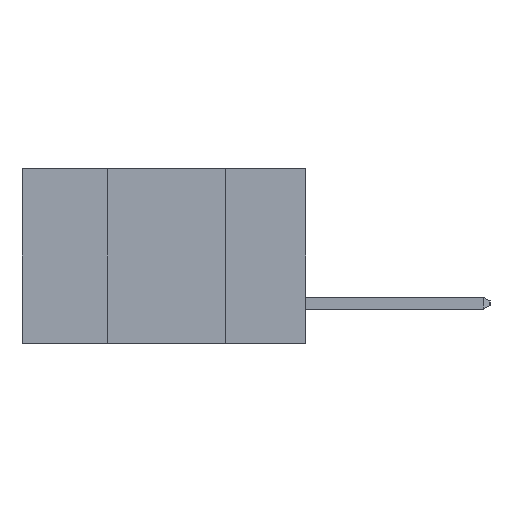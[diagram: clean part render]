
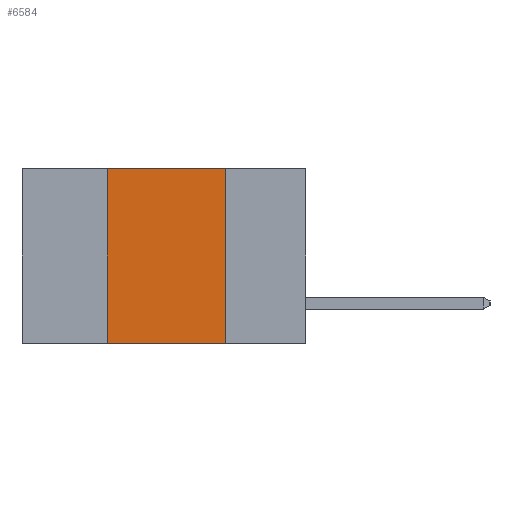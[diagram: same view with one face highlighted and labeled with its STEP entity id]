
A CAD part, left-side view. The second image highlights one B-rep face of the part: STEP entity #6584.
In plain terms, the highlighted planar face has unit normal (-1, 0, 0).
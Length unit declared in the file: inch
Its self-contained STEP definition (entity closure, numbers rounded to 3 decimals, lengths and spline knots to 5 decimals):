
#861 = VECTOR ( 'NONE', #4075, 39.37008 ) ;
#1150 = ORIENTED_EDGE ( 'NONE', *, *, #9027, .F. ) ;
#1529 = PLANE ( 'NONE',  #2654 ) ;
#1885 = LINE ( 'NONE', #4160, #7795 ) ;
#2454 = EDGE_CURVE ( 'NONE', #3641, #8773, #12826, .T. ) ;
#2654 = AXIS2_PLACEMENT_3D ( 'NONE', #12002, #5753, #13026 ) ;
#3023 = CARTESIAN_POINT ( 'NONE',  ( 0., 0.6, -0.37 ) ) ;
#3414 = EDGE_CURVE ( 'NONE', #5085, #8773, #9278, .T. ) ;
#3458 = FACE_OUTER_BOUND ( 'NONE', #7688, .T. ) ;
#3641 = VERTEX_POINT ( 'NONE', #5468 ) ;
#4075 = DIRECTION ( 'NONE',  ( 0., -1., 0. ) ) ;
#4160 = CARTESIAN_POINT ( 'NONE',  ( 0., 0.42, -0.37 ) ) ;
#4546 = VECTOR ( 'NONE', #10741, 39.37008 ) ;
#4553 = ORIENTED_EDGE ( 'NONE', *, *, #2454, .F. ) ;
#5043 = DIRECTION ( 'NONE',  ( 0., -1., 0. ) ) ;
#5085 = VERTEX_POINT ( 'NONE', #6775 ) ;
#5468 = CARTESIAN_POINT ( 'NONE',  ( 0., 0.17, 0. ) ) ;
#5485 = CARTESIAN_POINT ( 'NONE',  ( 0., 0.42, 0. ) ) ;
#5753 = DIRECTION ( 'NONE',  ( 1., 0., 0. ) ) ;
#6264 = VECTOR ( 'NONE', #5043, 39.37008 ) ;
#6425 = VERTEX_POINT ( 'NONE', #5485 ) ;
#6529 = ORIENTED_EDGE ( 'NONE', *, *, #3414, .T. ) ;
#6584 = ADVANCED_FACE ( 'NONE', ( #3458 ), #1529, .F. ) ;
#6775 = CARTESIAN_POINT ( 'NONE',  ( 0., 0.42, -0.37 ) ) ;
#7688 = EDGE_LOOP ( 'NONE', ( #4553, #8672, #1150, #6529 ) ) ;
#7795 = VECTOR ( 'NONE', #9427, 39.37008 ) ;
#8012 = CARTESIAN_POINT ( 'NONE',  ( 0., 0.17, -0.37 ) ) ;
#8672 = ORIENTED_EDGE ( 'NONE', *, *, #11115, .F. ) ;
#8773 = VERTEX_POINT ( 'NONE', #8012 ) ;
#9027 = EDGE_CURVE ( 'NONE', #5085, #6425, #1885, .T. ) ;
#9278 = LINE ( 'NONE', #3023, #861 ) ;
#9376 = LINE ( 'NONE', #10289, #6264 ) ;
#9427 = DIRECTION ( 'NONE',  ( 0., 0., 1. ) ) ;
#9692 = CARTESIAN_POINT ( 'NONE',  ( 0., 0.17, -0.37 ) ) ;
#10289 = CARTESIAN_POINT ( 'NONE',  ( 0., 0.6, 0. ) ) ;
#10741 = DIRECTION ( 'NONE',  ( 0., 0., -1. ) ) ;
#11115 = EDGE_CURVE ( 'NONE', #6425, #3641, #9376, .T. ) ;
#12002 = CARTESIAN_POINT ( 'NONE',  ( 0., 0.6, 0. ) ) ;
#12826 = LINE ( 'NONE', #9692, #4546 ) ;
#13026 = DIRECTION ( 'NONE',  ( 0., 0., -1. ) ) ;
